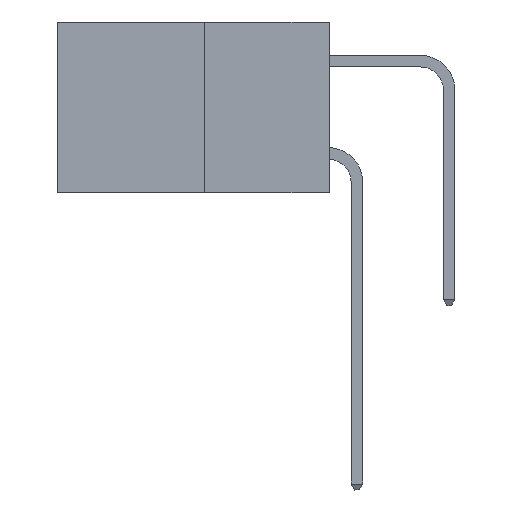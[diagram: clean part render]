
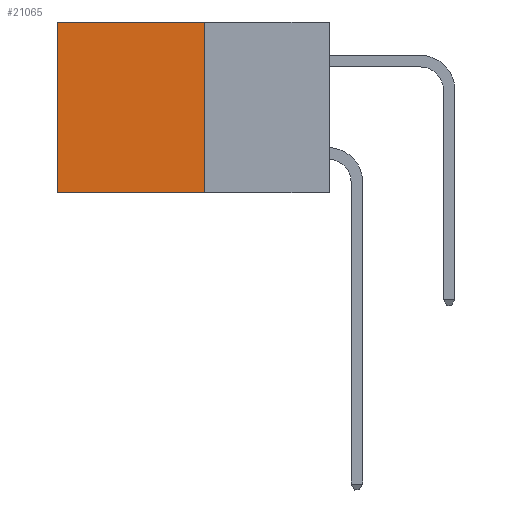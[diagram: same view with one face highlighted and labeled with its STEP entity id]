
A CAD part, left-side view. The second image highlights one B-rep face of the part: STEP entity #21065.
In plain terms, the highlighted planar face has unit normal (-1, 0, 0).
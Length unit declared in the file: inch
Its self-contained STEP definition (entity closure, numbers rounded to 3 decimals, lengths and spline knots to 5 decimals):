
#7 = EDGE_LOOP ( 'NONE', ( #23401, #1843, #25721, #25263 ) ) ;
#639 = CARTESIAN_POINT ( 'NONE',  ( 0.277, 0.27, -0.37 ) ) ;
#1843 = ORIENTED_EDGE ( 'NONE', *, *, #18930, .F. ) ;
#1992 = VECTOR ( 'NONE', #28393, 39.37008 ) ;
#2625 = FACE_OUTER_BOUND ( 'NONE', #7, .T. ) ;
#2845 = EDGE_CURVE ( 'NONE', #14328, #20112, #19794, .T. ) ;
#4165 = EDGE_CURVE ( 'NONE', #20112, #17415, #21059, .T. ) ;
#7036 = CARTESIAN_POINT ( 'NONE',  ( 0.277, 0.27, 0. ) ) ;
#7841 = AXIS2_PLACEMENT_3D ( 'NONE', #13150, #28534, #15412 ) ;
#9570 = CARTESIAN_POINT ( 'NONE',  ( 0.277, 0.59, 0. ) ) ;
#9677 = VECTOR ( 'NONE', #11764, 39.37008 ) ;
#11334 = VERTEX_POINT ( 'NONE', #24507 ) ;
#11764 = DIRECTION ( 'NONE',  ( 0., 1., 0. ) ) ;
#11957 = DIRECTION ( 'NONE',  ( 0., 0., -1. ) ) ;
#13150 = CARTESIAN_POINT ( 'NONE',  ( 0.277, 0.27, -0.37 ) ) ;
#13752 = EDGE_CURVE ( 'NONE', #14328, #11334, #20625, .T. ) ;
#14328 = VERTEX_POINT ( 'NONE', #7036 ) ;
#14758 = VECTOR ( 'NONE', #11957, 39.37008 ) ;
#15222 = VECTOR ( 'NONE', #21095, 39.37008 ) ;
#15412 = DIRECTION ( 'NONE',  ( 0., 0., -1. ) ) ;
#17048 = LINE ( 'NONE', #639, #9677 ) ;
#17415 = VERTEX_POINT ( 'NONE', #18120 ) ;
#18120 = CARTESIAN_POINT ( 'NONE',  ( 0.277, 0.59, -0.37 ) ) ;
#18930 = EDGE_CURVE ( 'NONE', #11334, #17415, #17048, .T. ) ;
#19306 = CARTESIAN_POINT ( 'NONE',  ( 0.277, 0.59, -0.37 ) ) ;
#19794 = LINE ( 'NONE', #28489, #1992 ) ;
#20112 = VERTEX_POINT ( 'NONE', #9570 ) ;
#20625 = LINE ( 'NONE', #20790, #14758 ) ;
#20790 = CARTESIAN_POINT ( 'NONE',  ( 0.277, 0.27, -0.37 ) ) ;
#21059 = LINE ( 'NONE', #19306, #15222 ) ;
#21065 = ADVANCED_FACE ( 'NONE', ( #2625 ), #21925, .F. ) ;
#21095 = DIRECTION ( 'NONE',  ( 0., 0., -1. ) ) ;
#21925 = PLANE ( 'NONE',  #7841 ) ;
#23401 = ORIENTED_EDGE ( 'NONE', *, *, #4165, .T. ) ;
#24507 = CARTESIAN_POINT ( 'NONE',  ( 0.277, 0.27, -0.37 ) ) ;
#25263 = ORIENTED_EDGE ( 'NONE', *, *, #2845, .T. ) ;
#25721 = ORIENTED_EDGE ( 'NONE', *, *, #13752, .F. ) ;
#28393 = DIRECTION ( 'NONE',  ( 0., 1., 0. ) ) ;
#28489 = CARTESIAN_POINT ( 'NONE',  ( 0.277, 0.27, 0. ) ) ;
#28534 = DIRECTION ( 'NONE',  ( 1., 0., 0. ) ) ;
